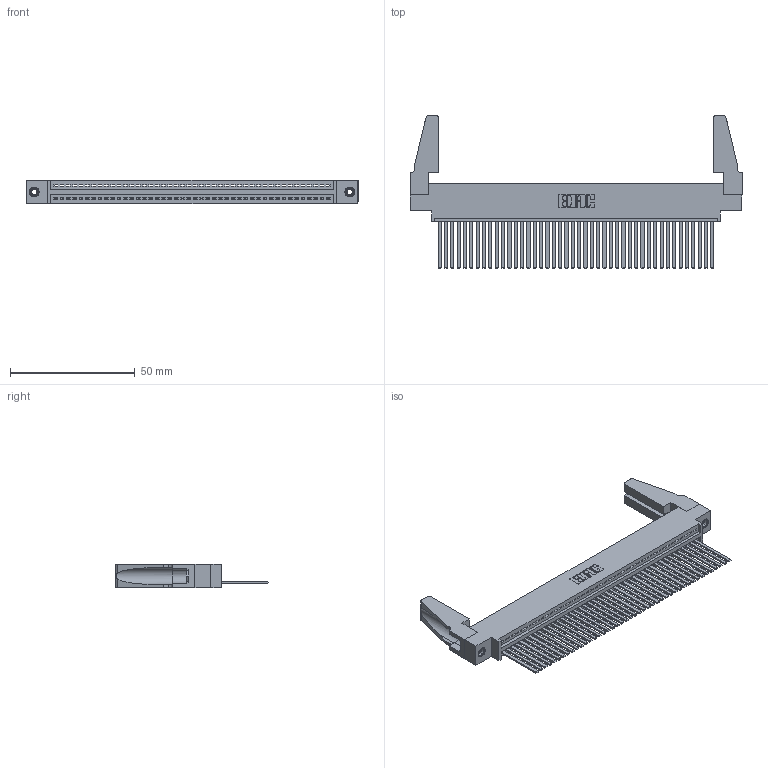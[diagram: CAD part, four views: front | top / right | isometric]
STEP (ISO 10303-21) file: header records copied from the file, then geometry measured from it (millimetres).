
FILE_DESCRIPTION (( 'STEP AP203' ), '1' );
FILE_NAME ('395-044-544-688.STEP', '2019-10-22T17:10:29', ( '' ), ( '' ), 'SwSTEP 2.0', 'SolidWorks 2016', '' );
FILE_SCHEMA (( 'CONFIG_CONTROL_DESIGN' ));
Length unit declared in the file: inch
Products named in the file (5): 345-292-001_345-293-144; 345-220-078_345-220-088; 395-044-544-688; 345 Part_0.170 Offset - 0.156 Dia-TH; 345-250-001_345-250-001-102
Assembly tree (49 placements, depth 2):
  395-044-544-688
    345 Part_0.170 Offset - 0.156 Dia-TH
    345-292-001_345-293-144  x44
    345-250-001_345-250-001-102  x2
    345-220-078_345-220-088  x2
Bounding box: 132.99 x 61.14 x 9.4 mm (x, y, z)
Volume: 16297 mm3; surface area: 22147.8 mm2
Topology: 49 solids, 49 shells, 2542 faces, 7619 edges, 5010 vertices
Faces by surface type: plane 1740, cylinder 786, cone 12, torus 4
Entity records: 34942 total; most frequent: CARTESIAN_POINT 6042, ORIENTED_EDGE 5980, DIRECTION 5278, EDGE_CURVE 2990, LINE 2644, VECTOR 2644, VERTEX_POINT 1986, AXIS2_PLACEMENT_3D 1317
